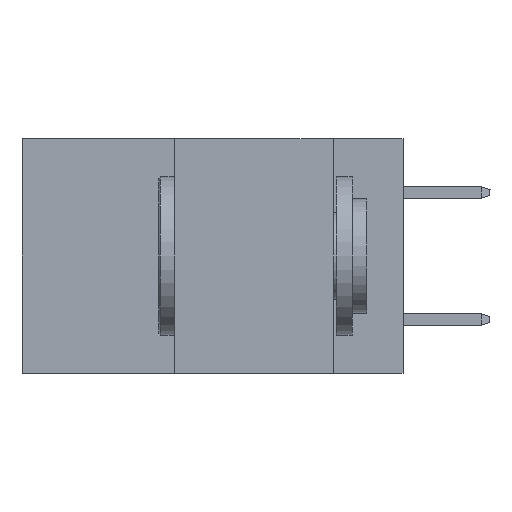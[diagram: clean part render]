
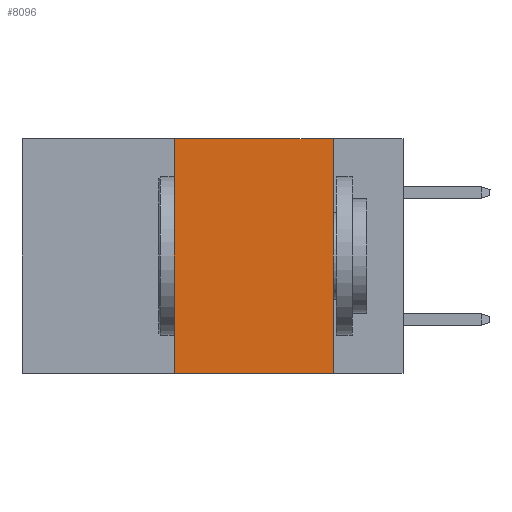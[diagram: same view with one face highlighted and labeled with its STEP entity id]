
A CAD part, left-side view. The second image highlights one B-rep face of the part: STEP entity #8096.
In plain terms, the highlighted planar face has unit normal (-1, 0, 0).
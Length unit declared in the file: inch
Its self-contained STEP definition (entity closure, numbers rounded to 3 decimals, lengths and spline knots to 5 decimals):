
#541 = FACE_OUTER_BOUND ( 'NONE', #6263, .T. ) ;
#1091 = LINE ( 'NONE', #16585, #10240 ) ;
#1191 = DIRECTION ( 'NONE',  ( 0., 0., 1. ) ) ;
#2027 = CARTESIAN_POINT ( 'NONE',  ( 0., 0.36, -0.37 ) ) ;
#2083 = PLANE ( 'NONE',  #6623 ) ;
#2302 = DIRECTION ( 'NONE',  ( 1., 0., 0. ) ) ;
#3065 = LINE ( 'NONE', #4344, #20524 ) ;
#4023 = CARTESIAN_POINT ( 'NONE',  ( 0., 0.6, 0. ) ) ;
#4344 = CARTESIAN_POINT ( 'NONE',  ( 0., 0.6, 0. ) ) ;
#6010 = ORIENTED_EDGE ( 'NONE', *, *, #8970, .T. ) ;
#6135 = EDGE_CURVE ( 'NONE', #17949, #10314, #9347, .T. ) ;
#6263 = EDGE_LOOP ( 'NONE', ( #19100, #20327, #10006, #6010 ) ) ;
#6623 = AXIS2_PLACEMENT_3D ( 'NONE', #4023, #2302, #9155 ) ;
#6656 = VECTOR ( 'NONE', #13191, 39.37008 ) ;
#7820 = LINE ( 'NONE', #17944, #6656 ) ;
#8041 = VERTEX_POINT ( 'NONE', #21042 ) ;
#8096 = ADVANCED_FACE ( 'NONE', ( #541 ), #2083, .F. ) ;
#8416 = VECTOR ( 'NONE', #12506, 39.37008 ) ;
#8932 = EDGE_CURVE ( 'NONE', #18055, #8041, #1091, .T. ) ;
#8970 = EDGE_CURVE ( 'NONE', #18055, #10314, #7820, .T. ) ;
#9155 = DIRECTION ( 'NONE',  ( 0., 0., -1. ) ) ;
#9347 = LINE ( 'NONE', #19674, #8416 ) ;
#9795 = CARTESIAN_POINT ( 'NONE',  ( 0., 0.11, 0. ) ) ;
#9928 = DIRECTION ( 'NONE',  ( 0., -1., 0. ) ) ;
#10006 = ORIENTED_EDGE ( 'NONE', *, *, #8932, .F. ) ;
#10240 = VECTOR ( 'NONE', #1191, 39.37008 ) ;
#10314 = VERTEX_POINT ( 'NONE', #20955 ) ;
#12506 = DIRECTION ( 'NONE',  ( 0., 0., -1. ) ) ;
#13191 = DIRECTION ( 'NONE',  ( 0., -1., 0. ) ) ;
#16585 = CARTESIAN_POINT ( 'NONE',  ( 0., 0.36, 0. ) ) ;
#17944 = CARTESIAN_POINT ( 'NONE',  ( 0., 0.6, -0.37 ) ) ;
#17949 = VERTEX_POINT ( 'NONE', #9795 ) ;
#18055 = VERTEX_POINT ( 'NONE', #2027 ) ;
#18666 = EDGE_CURVE ( 'NONE', #8041, #17949, #3065, .T. ) ;
#19100 = ORIENTED_EDGE ( 'NONE', *, *, #6135, .F. ) ;
#19674 = CARTESIAN_POINT ( 'NONE',  ( 0., 0.11, 0. ) ) ;
#20327 = ORIENTED_EDGE ( 'NONE', *, *, #18666, .F. ) ;
#20524 = VECTOR ( 'NONE', #9928, 39.37008 ) ;
#20955 = CARTESIAN_POINT ( 'NONE',  ( 0., 0.11, -0.37 ) ) ;
#21042 = CARTESIAN_POINT ( 'NONE',  ( 0., 0.36, 0. ) ) ;
